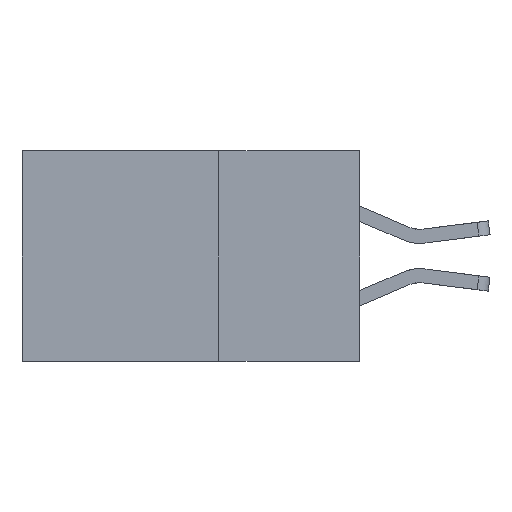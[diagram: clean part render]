
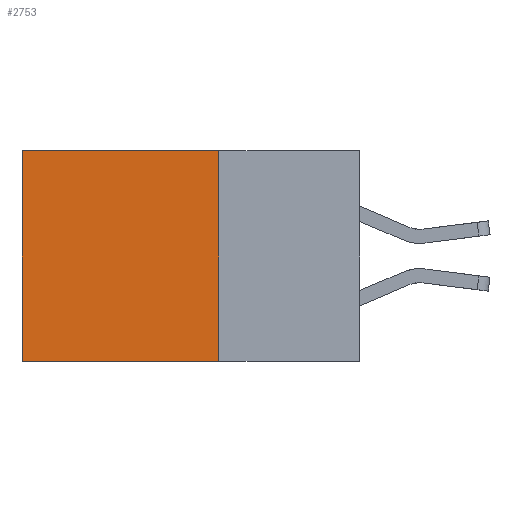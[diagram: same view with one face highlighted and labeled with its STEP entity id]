
A CAD part, left-side view. The second image highlights one B-rep face of the part: STEP entity #2753.
In plain terms, the highlighted planar face has unit normal (-1, 0, 0).
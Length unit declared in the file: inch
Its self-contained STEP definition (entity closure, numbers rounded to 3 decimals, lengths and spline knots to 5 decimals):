
#373 = VERTEX_POINT ( 'NONE', #5527 ) ;
#818 = LINE ( 'NONE', #2979, #4215 ) ;
#1232 = VECTOR ( 'NONE', #7505, 39.37008 ) ;
#1491 = VECTOR ( 'NONE', #4548, 39.37008 ) ;
#1652 = FACE_OUTER_BOUND ( 'NONE', #5110, .T. ) ;
#1756 = EDGE_CURVE ( 'NONE', #8771, #8208, #818, .T. ) ;
#2210 = DIRECTION ( 'NONE',  ( 0., 0., -1. ) ) ;
#2255 = PLANE ( 'NONE',  #9375 ) ;
#2295 = CARTESIAN_POINT ( 'NONE',  ( 0.2875, 0.25, 0. ) ) ;
#2670 = CARTESIAN_POINT ( 'NONE',  ( 0.2875, 0.6, -0.375 ) ) ;
#2753 = ADVANCED_FACE ( 'NONE', ( #1652 ), #2255, .F. ) ;
#2979 = CARTESIAN_POINT ( 'NONE',  ( 0.2875, 0.6, -0.375 ) ) ;
#3200 = VECTOR ( 'NONE', #9377, 39.37008 ) ;
#3760 = DIRECTION ( 'NONE',  ( 1., 0., 0. ) ) ;
#4177 = EDGE_CURVE ( 'NONE', #8644, #8771, #8078, .T. ) ;
#4215 = VECTOR ( 'NONE', #2210, 39.37008 ) ;
#4548 = DIRECTION ( 'NONE',  ( 0., 0., -1. ) ) ;
#4565 = CARTESIAN_POINT ( 'NONE',  ( 0.2875, 0.25, -0.375 ) ) ;
#4998 = LINE ( 'NONE', #7649, #1491 ) ;
#5110 = EDGE_LOOP ( 'NONE', ( #6587, #8999, #9607, #10004 ) ) ;
#5332 = EDGE_CURVE ( 'NONE', #373, #8208, #9273, .T. ) ;
#5527 = CARTESIAN_POINT ( 'NONE',  ( 0.2875, 0.25, -0.375 ) ) ;
#5708 = CARTESIAN_POINT ( 'NONE',  ( 0.2875, 0.25, 0. ) ) ;
#6587 = ORIENTED_EDGE ( 'NONE', *, *, #1756, .T. ) ;
#6670 = CARTESIAN_POINT ( 'NONE',  ( 0.2875, 0.25, -0.375 ) ) ;
#7505 = DIRECTION ( 'NONE',  ( 0., 1., 0. ) ) ;
#7649 = CARTESIAN_POINT ( 'NONE',  ( 0.2875, 0.25, -0.375 ) ) ;
#8078 = LINE ( 'NONE', #5708, #3200 ) ;
#8208 = VERTEX_POINT ( 'NONE', #2670 ) ;
#8644 = VERTEX_POINT ( 'NONE', #2295 ) ;
#8771 = VERTEX_POINT ( 'NONE', #8796 ) ;
#8796 = CARTESIAN_POINT ( 'NONE',  ( 0.2875, 0.6, 0. ) ) ;
#8999 = ORIENTED_EDGE ( 'NONE', *, *, #5332, .F. ) ;
#9273 = LINE ( 'NONE', #6670, #1232 ) ;
#9375 = AXIS2_PLACEMENT_3D ( 'NONE', #4565, #3760, #10013 ) ;
#9377 = DIRECTION ( 'NONE',  ( 0., 1., 0. ) ) ;
#9607 = ORIENTED_EDGE ( 'NONE', *, *, #9821, .F. ) ;
#9821 = EDGE_CURVE ( 'NONE', #8644, #373, #4998, .T. ) ;
#10004 = ORIENTED_EDGE ( 'NONE', *, *, #4177, .T. ) ;
#10013 = DIRECTION ( 'NONE',  ( 0., 0., -1. ) ) ;
